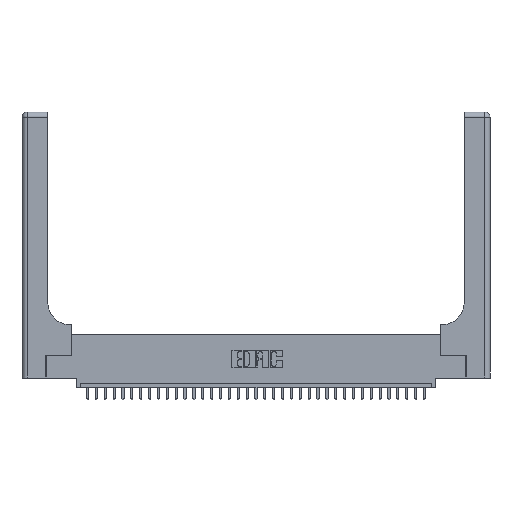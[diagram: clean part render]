
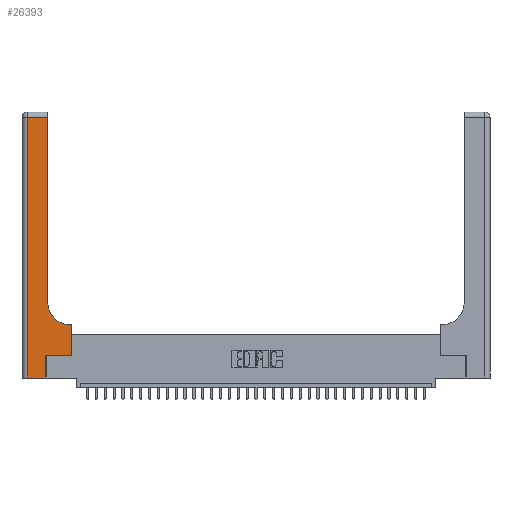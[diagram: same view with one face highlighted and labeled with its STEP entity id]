
A CAD part, top view. The second image highlights one B-rep face of the part: STEP entity #26393.
In plain terms, the highlighted planar face has unit normal (0, 0, 1).
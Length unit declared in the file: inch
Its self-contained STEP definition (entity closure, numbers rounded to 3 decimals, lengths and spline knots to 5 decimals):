
#77 = CARTESIAN_POINT ( 'NONE',  ( 0.2915, 3., 0.37 ) ) ;
#97 = LINE ( 'NONE', #29646, #14961 ) ;
#156 = LINE ( 'NONE', #31589, #12940 ) ;
#1956 = ORIENTED_EDGE ( 'NONE', *, *, #20538, .T. ) ;
#2204 = ORIENTED_EDGE ( 'NONE', *, *, #16888, .T. ) ;
#2484 = LINE ( 'NONE', #77, #21550 ) ;
#3774 = CARTESIAN_POINT ( 'NONE',  ( 0.5585, 0.25, 0.37 ) ) ;
#4653 = FACE_OUTER_BOUND ( 'NONE', #16578, .T. ) ;
#5610 = ORIENTED_EDGE ( 'NONE', *, *, #28303, .T. ) ;
#5742 = DIRECTION ( 'NONE',  ( -1., 0., 0. ) ) ;
#6142 = DIRECTION ( 'NONE',  ( 1., 0., 0. ) ) ;
#6248 = ORIENTED_EDGE ( 'NONE', *, *, #23385, .T. ) ;
#6371 = EDGE_CURVE ( 'NONE', #17953, #28697, #11401, .T. ) ;
#7085 = CARTESIAN_POINT ( 'NONE',  ( 0.269, 0., 0.37 ) ) ;
#7505 = CARTESIAN_POINT ( 'NONE',  ( 0.5415, 0.85, 0.37 ) ) ;
#8078 = DIRECTION ( 'NONE',  ( 0., 1., 0. ) ) ;
#8147 = CARTESIAN_POINT ( 'NONE',  ( 0.5415, 0.6, 0.37 ) ) ;
#8859 = VECTOR ( 'NONE', #23577, 39.37008 ) ;
#10208 = CARTESIAN_POINT ( 'NONE',  ( 0.2915, 0.85, 0.37 ) ) ;
#10234 = ORIENTED_EDGE ( 'NONE', *, *, #24654, .T. ) ;
#10539 = ORIENTED_EDGE ( 'NONE', *, *, #16020, .T. ) ;
#11359 = ORIENTED_EDGE ( 'NONE', *, *, #23753, .T. ) ;
#11401 = LINE ( 'NONE', #27753, #19426 ) ;
#11431 = DIRECTION ( 'NONE',  ( 0., 1., 0. ) ) ;
#12940 = VECTOR ( 'NONE', #31107, 39.37008 ) ;
#13545 = LINE ( 'NONE', #27125, #34297 ) ;
#13561 = DIRECTION ( 'NONE',  ( -1., 0., 0. ) ) ;
#14961 = VECTOR ( 'NONE', #13561, 39.37008 ) ;
#15216 = CARTESIAN_POINT ( 'NONE',  ( 0.2915, 2.94, 0.37 ) ) ;
#16020 = EDGE_CURVE ( 'NONE', #25152, #18785, #2484, .T. ) ;
#16141 = AXIS2_PLACEMENT_3D ( 'NONE', #23235, #32431, #5742 ) ;
#16326 = CIRCLE ( 'NONE', #20621, 0.25 ) ;
#16578 = EDGE_LOOP ( 'NONE', ( #10539, #10234, #27580, #34498, #5610, #11359, #2204, #1956, #6248 ) ) ;
#16888 = EDGE_CURVE ( 'NONE', #34216, #25124, #26122, .T. ) ;
#17138 = VECTOR ( 'NONE', #20905, 39.37008 ) ;
#17953 = VERTEX_POINT ( 'NONE', #31634 ) ;
#18584 = DIRECTION ( 'NONE',  ( 1., 0., 0. ) ) ;
#18785 = VERTEX_POINT ( 'NONE', #15216 ) ;
#19426 = VECTOR ( 'NONE', #6142, 39.37008 ) ;
#20377 = VERTEX_POINT ( 'NONE', #29935 ) ;
#20538 = EDGE_CURVE ( 'NONE', #25124, #24033, #13545, .T. ) ;
#20621 = AXIS2_PLACEMENT_3D ( 'NONE', #7505, #26395, #18584 ) ;
#20905 = DIRECTION ( 'NONE',  ( 0., 1., 0. ) ) ;
#21550 = VECTOR ( 'NONE', #8078, 39.37008 ) ;
#22131 = PLANE ( 'NONE',  #16141 ) ;
#22225 = CARTESIAN_POINT ( 'NONE',  ( 0.269, 0., 0.37 ) ) ;
#22868 = CARTESIAN_POINT ( 'NONE',  ( 0.5585, 0.25, 0.37 ) ) ;
#23235 = CARTESIAN_POINT ( 'NONE',  ( 0., 3., 0.37 ) ) ;
#23328 = CARTESIAN_POINT ( 'NONE',  ( 0.06, 3., 0.37 ) ) ;
#23385 = EDGE_CURVE ( 'NONE', #24033, #25152, #16326, .T. ) ;
#23577 = DIRECTION ( 'NONE',  ( 0., -1., 0. ) ) ;
#23753 = EDGE_CURVE ( 'NONE', #20377, #34216, #156, .T. ) ;
#23804 = VERTEX_POINT ( 'NONE', #34178 ) ;
#24033 = VERTEX_POINT ( 'NONE', #8147 ) ;
#24403 = VECTOR ( 'NONE', #11431, 39.37008 ) ;
#24654 = EDGE_CURVE ( 'NONE', #18785, #23804, #97, .T. ) ;
#25124 = VERTEX_POINT ( 'NONE', #30437 ) ;
#25152 = VERTEX_POINT ( 'NONE', #10208 ) ;
#26083 = EDGE_CURVE ( 'NONE', #23804, #17953, #26693, .T. ) ;
#26122 = LINE ( 'NONE', #3774, #24403 ) ;
#26393 = ADVANCED_FACE ( 'NONE', ( #4653 ), #22131, .F. ) ;
#26395 = DIRECTION ( 'NONE',  ( 0., 0., -1. ) ) ;
#26693 = LINE ( 'NONE', #23328, #8859 ) ;
#27125 = CARTESIAN_POINT ( 'NONE',  ( 0.2915, 0.6, 0.37 ) ) ;
#27580 = ORIENTED_EDGE ( 'NONE', *, *, #26083, .T. ) ;
#27753 = CARTESIAN_POINT ( 'NONE',  ( 0., 0., 0.37 ) ) ;
#28303 = EDGE_CURVE ( 'NONE', #28697, #20377, #34969, .T. ) ;
#28697 = VERTEX_POINT ( 'NONE', #22225 ) ;
#29646 = CARTESIAN_POINT ( 'NONE',  ( 0., 2.94, 0.37 ) ) ;
#29848 = DIRECTION ( 'NONE',  ( -1., 0., 0. ) ) ;
#29935 = CARTESIAN_POINT ( 'NONE',  ( 0.269, 0.25, 0.37 ) ) ;
#30437 = CARTESIAN_POINT ( 'NONE',  ( 0.5585, 0.6, 0.37 ) ) ;
#31107 = DIRECTION ( 'NONE',  ( 1., 0., 0. ) ) ;
#31589 = CARTESIAN_POINT ( 'NONE',  ( 0.269, 0.25, 0.37 ) ) ;
#31634 = CARTESIAN_POINT ( 'NONE',  ( 0.06, 0., 0.37 ) ) ;
#32431 = DIRECTION ( 'NONE',  ( 0., 0., -1. ) ) ;
#34178 = CARTESIAN_POINT ( 'NONE',  ( 0.06, 2.94, 0.37 ) ) ;
#34216 = VERTEX_POINT ( 'NONE', #22868 ) ;
#34297 = VECTOR ( 'NONE', #29848, 39.37008 ) ;
#34498 = ORIENTED_EDGE ( 'NONE', *, *, #6371, .T. ) ;
#34969 = LINE ( 'NONE', #7085, #17138 ) ;
